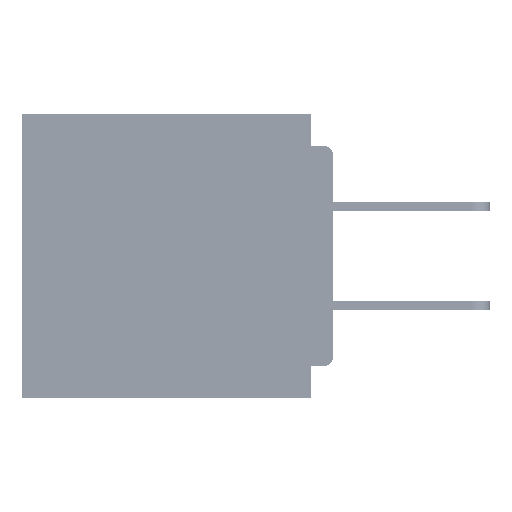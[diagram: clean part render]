
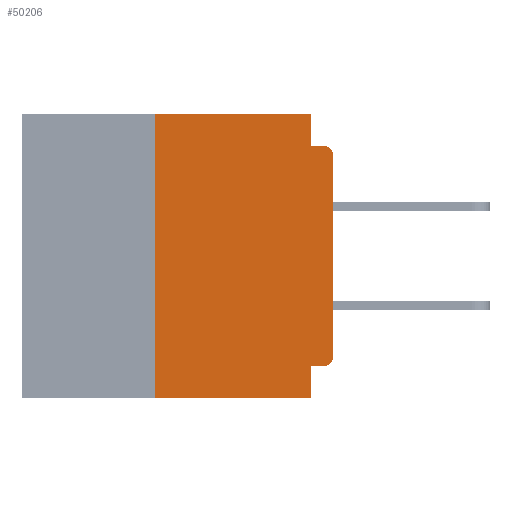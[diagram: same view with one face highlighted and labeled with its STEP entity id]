
A CAD part, left-side view. The second image highlights one B-rep face of the part: STEP entity #50206.
In plain terms, the highlighted planar face has unit normal (-1, 0, 0).
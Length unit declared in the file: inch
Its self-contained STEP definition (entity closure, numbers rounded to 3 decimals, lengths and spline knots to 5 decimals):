
#73 = ORIENTED_EDGE ( 'NONE', *, *, #59666, .F. ) ;
#117 = EDGE_CURVE ( 'NONE', #28982, #53349, #18122, .T. ) ;
#676 = EDGE_CURVE ( 'NONE', #53656, #53349, #23345, .T. ) ;
#1348 = ORIENTED_EDGE ( 'NONE', *, *, #3035, .T. ) ;
#2035 = LINE ( 'NONE', #41335, #26395 ) ;
#3035 = EDGE_CURVE ( 'NONE', #26436, #24662, #41257, .T. ) ;
#3149 = CARTESIAN_POINT ( 'NONE',  ( 0., 0., -0.045 ) ) ;
#3222 = CARTESIAN_POINT ( 'NONE',  ( 0., 0.015, -0.045 ) ) ;
#3645 = VECTOR ( 'NONE', #19292, 39.37008 ) ;
#4514 = FACE_OUTER_BOUND ( 'NONE', #44449, .T. ) ;
#6802 = LINE ( 'NONE', #3149, #18206 ) ;
#8188 = CARTESIAN_POINT ( 'NONE',  ( 0., 0.437, 0. ) ) ;
#8847 = DIRECTION ( 'NONE',  ( -1., 0., 0. ) ) ;
#9507 = VERTEX_POINT ( 'NONE', #3222 ) ;
#9701 = ORIENTED_EDGE ( 'NONE', *, *, #44072, .F. ) ;
#11376 = CIRCLE ( 'NONE', #17784, 0.015 ) ;
#11410 = CARTESIAN_POINT ( 'NONE',  ( 0., 0., 0. ) ) ;
#12180 = CARTESIAN_POINT ( 'NONE',  ( 0., 0.015, -0.355 ) ) ;
#12542 = DIRECTION ( 'NONE',  ( -1., 0., 0. ) ) ;
#12565 = LINE ( 'NONE', #30797, #62395 ) ;
#14895 = ORIENTED_EDGE ( 'NONE', *, *, #26534, .F. ) ;
#15055 = VERTEX_POINT ( 'NONE', #55098 ) ;
#15923 = ORIENTED_EDGE ( 'NONE', *, *, #117, .T. ) ;
#16283 = CARTESIAN_POINT ( 'NONE',  ( 0., 0.031, 0. ) ) ;
#16363 = CARTESIAN_POINT ( 'NONE',  ( 0., 0.437, -0.4 ) ) ;
#17784 = AXIS2_PLACEMENT_3D ( 'NONE', #41614, #12542, #46466 ) ;
#18122 = LINE ( 'NONE', #16363, #3645 ) ;
#18206 = VECTOR ( 'NONE', #61288, 39.37008 ) ;
#18298 = DIRECTION ( 'NONE',  ( 1., 0., 0. ) ) ;
#19292 = DIRECTION ( 'NONE',  ( 0., -1., 0. ) ) ;
#21082 = LINE ( 'NONE', #49477, #32423 ) ;
#22036 = DIRECTION ( 'NONE',  ( 0., 1., 0. ) ) ;
#22213 = CARTESIAN_POINT ( 'NONE',  ( 0., 0., -0.34 ) ) ;
#22478 = ORIENTED_EDGE ( 'NONE', *, *, #38958, .F. ) ;
#23345 = LINE ( 'NONE', #42359, #49091 ) ;
#23390 = ORIENTED_EDGE ( 'NONE', *, *, #46288, .F. ) ;
#24662 = VERTEX_POINT ( 'NONE', #35219 ) ;
#25366 = DIRECTION ( 'NONE',  ( 0., 0., 1. ) ) ;
#26395 = VECTOR ( 'NONE', #22036, 39.37008 ) ;
#26436 = VERTEX_POINT ( 'NONE', #22213 ) ;
#26534 = EDGE_CURVE ( 'NONE', #15055, #37480, #32439, .T. ) ;
#26705 = ORIENTED_EDGE ( 'NONE', *, *, #676, .F. ) ;
#28982 = VERTEX_POINT ( 'NONE', #57960 ) ;
#29853 = VECTOR ( 'NONE', #45338, 39.37008 ) ;
#30674 = AXIS2_PLACEMENT_3D ( 'NONE', #37871, #8847, #42784 ) ;
#30797 = CARTESIAN_POINT ( 'NONE',  ( 0., 0.031, 0. ) ) ;
#32423 = VECTOR ( 'NONE', #25366, 39.37008 ) ;
#32439 = LINE ( 'NONE', #8188, #56615 ) ;
#34292 = VERTEX_POINT ( 'NONE', #12180 ) ;
#35219 = CARTESIAN_POINT ( 'NONE',  ( 0., 0., -0.06 ) ) ;
#37480 = VERTEX_POINT ( 'NONE', #16283 ) ;
#37871 = CARTESIAN_POINT ( 'NONE',  ( 0., 0.015, -0.06 ) ) ;
#38734 = CARTESIAN_POINT ( 'NONE',  ( 0., 0.031, -0.355 ) ) ;
#38958 = EDGE_CURVE ( 'NONE', #34292, #53656, #2035, .T. ) ;
#39472 = VERTEX_POINT ( 'NONE', #56003 ) ;
#41257 = LINE ( 'NONE', #11410, #29853 ) ;
#41327 = CARTESIAN_POINT ( 'NONE',  ( 0., 0.031, -0.4 ) ) ;
#41335 = CARTESIAN_POINT ( 'NONE',  ( 0., 0., -0.355 ) ) ;
#41614 = CARTESIAN_POINT ( 'NONE',  ( 0., 0.015, -0.34 ) ) ;
#42148 = DIRECTION ( 'NONE',  ( 0., 0., -1. ) ) ;
#42359 = CARTESIAN_POINT ( 'NONE',  ( 0., 0.031, -0.4 ) ) ;
#42481 = PLANE ( 'NONE',  #56119 ) ;
#42784 = DIRECTION ( 'NONE',  ( 0., 0., -1. ) ) ;
#43988 = EDGE_CURVE ( 'NONE', #34292, #26436, #11376, .T. ) ;
#44072 = EDGE_CURVE ( 'NONE', #39472, #9507, #6802, .T. ) ;
#44449 = EDGE_LOOP ( 'NONE', ( #1348, #45589, #9701, #23390, #14895, #73, #15923, #26705, #22478, #60333 ) ) ;
#45338 = DIRECTION ( 'NONE',  ( 0., 0., 1. ) ) ;
#45589 = ORIENTED_EDGE ( 'NONE', *, *, #51721, .T. ) ;
#46288 = EDGE_CURVE ( 'NONE', #37480, #39472, #12565, .T. ) ;
#46466 = DIRECTION ( 'NONE',  ( 0., 0., -1. ) ) ;
#47162 = DIRECTION ( 'NONE',  ( 0., -1., 0. ) ) ;
#47310 = CARTESIAN_POINT ( 'NONE',  ( 0., 0.437, 0. ) ) ;
#49091 = VECTOR ( 'NONE', #42148, 39.37008 ) ;
#49477 = CARTESIAN_POINT ( 'NONE',  ( 0., 0.25, -0.4 ) ) ;
#50206 = ADVANCED_FACE ( 'NONE', ( #4514 ), #42481, .F. ) ;
#51721 = EDGE_CURVE ( 'NONE', #24662, #9507, #59558, .T. ) ;
#52150 = DIRECTION ( 'NONE',  ( 0., 0., -1. ) ) ;
#53349 = VERTEX_POINT ( 'NONE', #41327 ) ;
#53656 = VERTEX_POINT ( 'NONE', #38734 ) ;
#55095 = DIRECTION ( 'NONE',  ( 0., 0., -1. ) ) ;
#55098 = CARTESIAN_POINT ( 'NONE',  ( 0., 0.25, 0. ) ) ;
#56003 = CARTESIAN_POINT ( 'NONE',  ( 0., 0.031, -0.045 ) ) ;
#56119 = AXIS2_PLACEMENT_3D ( 'NONE', #47310, #18298, #52150 ) ;
#56615 = VECTOR ( 'NONE', #47162, 39.37008 ) ;
#57960 = CARTESIAN_POINT ( 'NONE',  ( 0., 0.25, -0.4 ) ) ;
#59558 = CIRCLE ( 'NONE', #30674, 0.015 ) ;
#59666 = EDGE_CURVE ( 'NONE', #28982, #15055, #21082, .T. ) ;
#60333 = ORIENTED_EDGE ( 'NONE', *, *, #43988, .T. ) ;
#61288 = DIRECTION ( 'NONE',  ( 0., -1., 0. ) ) ;
#62395 = VECTOR ( 'NONE', #55095, 39.37008 ) ;
